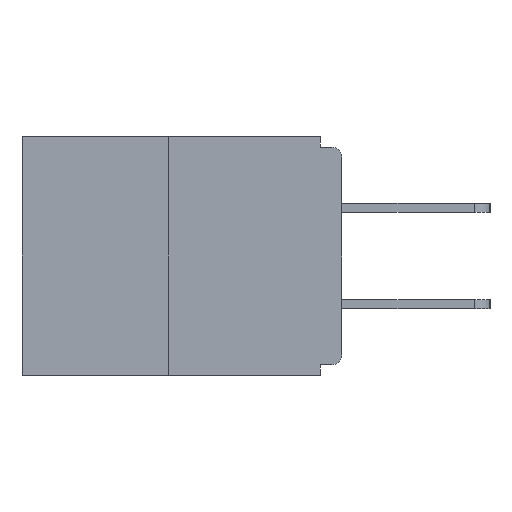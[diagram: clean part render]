
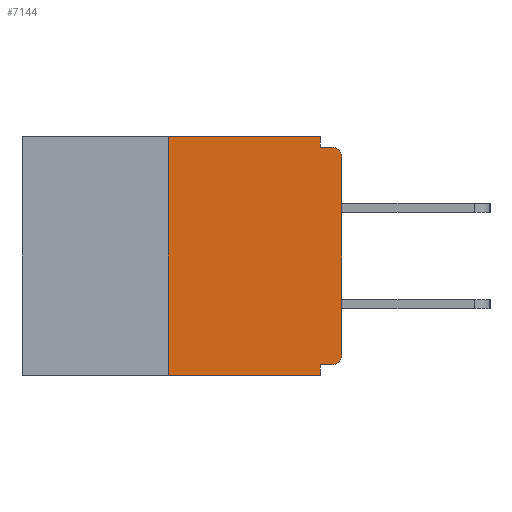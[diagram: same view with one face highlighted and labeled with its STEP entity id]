
A CAD part, left-side view. The second image highlights one B-rep face of the part: STEP entity #7144.
In plain terms, the highlighted planar face has unit normal (-1, 0, 0).
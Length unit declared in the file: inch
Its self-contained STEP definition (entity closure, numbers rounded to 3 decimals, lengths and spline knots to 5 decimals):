
#196 = ORIENTED_EDGE ( 'NONE', *, *, #11260, .F. ) ;
#305 = VECTOR ( 'NONE', #2225, 39.37008 ) ;
#327 = DIRECTION ( 'NONE',  ( 0., 0., -1. ) ) ;
#334 = EDGE_CURVE ( 'NONE', #8543, #12090, #6795, .T. ) ;
#344 = DIRECTION ( 'NONE',  ( 0., 0., -1. ) ) ;
#551 = PLANE ( 'NONE',  #851 ) ;
#851 = AXIS2_PLACEMENT_3D ( 'NONE', #16681, #1788, #327 ) ;
#856 = DIRECTION ( 'NONE',  ( -1., 0., 0. ) ) ;
#1093 = CARTESIAN_POINT ( 'NONE',  ( 0., 0.015, -0.313 ) ) ;
#1483 = EDGE_CURVE ( 'NONE', #5490, #8543, #13920, .T. ) ;
#1575 = ORIENTED_EDGE ( 'NONE', *, *, #1483, .F. ) ;
#1735 = CIRCLE ( 'NONE', #9668, 0.015 ) ;
#1788 = DIRECTION ( 'NONE',  ( 1., 0., 0. ) ) ;
#1845 = LINE ( 'NONE', #13514, #7350 ) ;
#2049 = CARTESIAN_POINT ( 'NONE',  ( 0., 0.031, -0.343 ) ) ;
#2205 = EDGE_CURVE ( 'NONE', #17373, #8934, #13063, .T. ) ;
#2225 = DIRECTION ( 'NONE',  ( 0., -1., 0. ) ) ;
#2248 = LINE ( 'NONE', #11230, #16202 ) ;
#2373 = DIRECTION ( 'NONE',  ( 0., 0., -1. ) ) ;
#2503 = EDGE_CURVE ( 'NONE', #9184, #5490, #1845, .T. ) ;
#2828 = ORIENTED_EDGE ( 'NONE', *, *, #2503, .F. ) ;
#3015 = ORIENTED_EDGE ( 'NONE', *, *, #334, .F. ) ;
#3094 = CARTESIAN_POINT ( 'NONE',  ( 0., 0.25, 0. ) ) ;
#3678 = CIRCLE ( 'NONE', #4553, 0.015 ) ;
#3822 = VERTEX_POINT ( 'NONE', #7275 ) ;
#4178 = VECTOR ( 'NONE', #8194, 39.37008 ) ;
#4209 = CARTESIAN_POINT ( 'NONE',  ( 0., 0.031, 0. ) ) ;
#4218 = EDGE_LOOP ( 'NONE', ( #2828, #196, #10113, #16554, #15680, #7470, #5092, #7024, #3015, #1575 ) ) ;
#4553 = AXIS2_PLACEMENT_3D ( 'NONE', #1093, #856, #6309 ) ;
#4597 = CARTESIAN_POINT ( 'NONE',  ( 0., 0.031, -0.015 ) ) ;
#4672 = EDGE_CURVE ( 'NONE', #9815, #17373, #3678, .T. ) ;
#5092 = ORIENTED_EDGE ( 'NONE', *, *, #2205, .T. ) ;
#5212 = EDGE_CURVE ( 'NONE', #8934, #12090, #1735, .T. ) ;
#5373 = LINE ( 'NONE', #14093, #305 ) ;
#5490 = VERTEX_POINT ( 'NONE', #9394 ) ;
#6249 = CARTESIAN_POINT ( 'NONE',  ( 0., 0.015, -0.015 ) ) ;
#6309 = DIRECTION ( 'NONE',  ( 0., 0., -1. ) ) ;
#6324 = CARTESIAN_POINT ( 'NONE',  ( 0., 0., -0.015 ) ) ;
#6348 = CARTESIAN_POINT ( 'NONE',  ( 0., 0.031, -0.328 ) ) ;
#6795 = LINE ( 'NONE', #6324, #11001 ) ;
#7024 = ORIENTED_EDGE ( 'NONE', *, *, #5212, .T. ) ;
#7144 = ADVANCED_FACE ( 'NONE', ( #11146 ), #551, .F. ) ;
#7275 = CARTESIAN_POINT ( 'NONE',  ( 0., 0.25, -0.343 ) ) ;
#7350 = VECTOR ( 'NONE', #7932, 39.37008 ) ;
#7470 = ORIENTED_EDGE ( 'NONE', *, *, #4672, .T. ) ;
#7832 = VECTOR ( 'NONE', #16288, 39.37008 ) ;
#7932 = DIRECTION ( 'NONE',  ( 0., -1., 0. ) ) ;
#8194 = DIRECTION ( 'NONE',  ( 0., 0., 1. ) ) ;
#8543 = VERTEX_POINT ( 'NONE', #4597 ) ;
#8833 = DIRECTION ( 'NONE',  ( 0., 0., 1. ) ) ;
#8934 = VERTEX_POINT ( 'NONE', #9441 ) ;
#9155 = LINE ( 'NONE', #15557, #14849 ) ;
#9184 = VERTEX_POINT ( 'NONE', #3094 ) ;
#9394 = CARTESIAN_POINT ( 'NONE',  ( 0., 0.031, 0. ) ) ;
#9441 = CARTESIAN_POINT ( 'NONE',  ( 0., 0., -0.03 ) ) ;
#9668 = AXIS2_PLACEMENT_3D ( 'NONE', #15800, #16032, #2373 ) ;
#9815 = VERTEX_POINT ( 'NONE', #14089 ) ;
#10113 = ORIENTED_EDGE ( 'NONE', *, *, #10737, .T. ) ;
#10129 = DIRECTION ( 'NONE',  ( 0., 1., 0. ) ) ;
#10652 = EDGE_CURVE ( 'NONE', #17135, #13600, #15958, .T. ) ;
#10737 = EDGE_CURVE ( 'NONE', #3822, #13600, #5373, .T. ) ;
#11001 = VECTOR ( 'NONE', #13092, 39.37008 ) ;
#11146 = FACE_OUTER_BOUND ( 'NONE', #4218, .T. ) ;
#11230 = CARTESIAN_POINT ( 'NONE',  ( 0., 0., -0.328 ) ) ;
#11260 = EDGE_CURVE ( 'NONE', #3822, #9184, #9155, .T. ) ;
#12090 = VERTEX_POINT ( 'NONE', #6249 ) ;
#12287 = EDGE_CURVE ( 'NONE', #9815, #17135, #2248, .T. ) ;
#12331 = CARTESIAN_POINT ( 'NONE',  ( 0., 0., -0.313 ) ) ;
#12340 = VECTOR ( 'NONE', #344, 39.37008 ) ;
#13063 = LINE ( 'NONE', #13639, #4178 ) ;
#13092 = DIRECTION ( 'NONE',  ( 0., -1., 0. ) ) ;
#13514 = CARTESIAN_POINT ( 'NONE',  ( 0., 0.46, 0. ) ) ;
#13600 = VERTEX_POINT ( 'NONE', #2049 ) ;
#13639 = CARTESIAN_POINT ( 'NONE',  ( 0., 0., 0. ) ) ;
#13920 = LINE ( 'NONE', #4209, #7832 ) ;
#14089 = CARTESIAN_POINT ( 'NONE',  ( 0., 0.015, -0.328 ) ) ;
#14093 = CARTESIAN_POINT ( 'NONE',  ( 0., 0.46, -0.343 ) ) ;
#14849 = VECTOR ( 'NONE', #8833, 39.37008 ) ;
#15167 = CARTESIAN_POINT ( 'NONE',  ( 0., 0.031, -0.343 ) ) ;
#15557 = CARTESIAN_POINT ( 'NONE',  ( 0., 0.25, 0. ) ) ;
#15680 = ORIENTED_EDGE ( 'NONE', *, *, #12287, .F. ) ;
#15800 = CARTESIAN_POINT ( 'NONE',  ( 0., 0.015, -0.03 ) ) ;
#15958 = LINE ( 'NONE', #15167, #12340 ) ;
#16032 = DIRECTION ( 'NONE',  ( -1., 0., 0. ) ) ;
#16202 = VECTOR ( 'NONE', #10129, 39.37008 ) ;
#16288 = DIRECTION ( 'NONE',  ( 0., 0., -1. ) ) ;
#16554 = ORIENTED_EDGE ( 'NONE', *, *, #10652, .F. ) ;
#16681 = CARTESIAN_POINT ( 'NONE',  ( 0., 0.46, 0. ) ) ;
#17135 = VERTEX_POINT ( 'NONE', #6348 ) ;
#17373 = VERTEX_POINT ( 'NONE', #12331 ) ;
